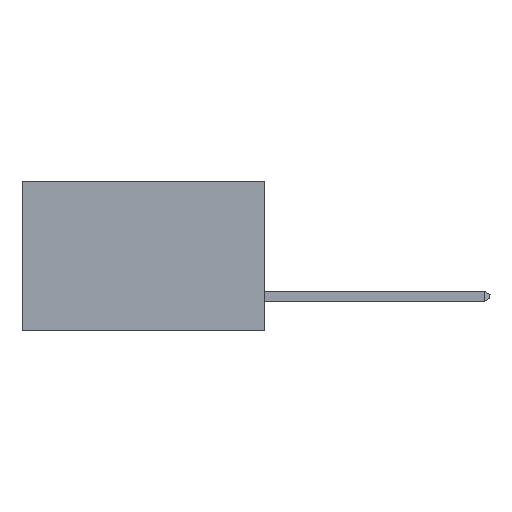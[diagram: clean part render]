
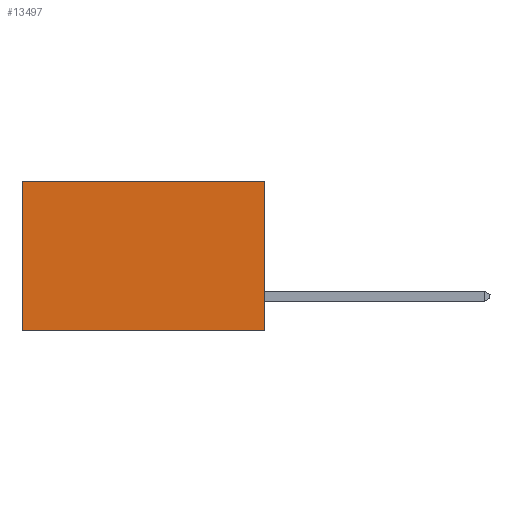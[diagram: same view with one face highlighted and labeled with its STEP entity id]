
A CAD part, left-side view. The second image highlights one B-rep face of the part: STEP entity #13497.
In plain terms, the highlighted planar face has unit normal (-1, 0, 0).
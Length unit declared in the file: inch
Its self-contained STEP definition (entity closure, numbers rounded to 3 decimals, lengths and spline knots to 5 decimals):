
#767 = VECTOR ( 'NONE', #15023, 39.37008 ) ;
#2367 = EDGE_CURVE ( 'NONE', #17266, #6237, #12811, .T. ) ;
#2376 = DIRECTION ( 'NONE',  ( 0., 0., -1. ) ) ;
#2412 = EDGE_CURVE ( 'NONE', #11081, #6237, #20683, .T. ) ;
#2813 = VERTEX_POINT ( 'NONE', #7000 ) ;
#3855 = CARTESIAN_POINT ( 'NONE',  ( 0.298, 0., 0. ) ) ;
#5524 = VECTOR ( 'NONE', #17310, 39.37008 ) ;
#5639 = CARTESIAN_POINT ( 'NONE',  ( 0.298, 0., 0. ) ) ;
#6237 = VERTEX_POINT ( 'NONE', #21857 ) ;
#6766 = EDGE_CURVE ( 'NONE', #2813, #17266, #20500, .T. ) ;
#7000 = CARTESIAN_POINT ( 'NONE',  ( 0.298, 0., 0. ) ) ;
#7264 = VECTOR ( 'NONE', #2376, 39.37008 ) ;
#7351 = EDGE_LOOP ( 'NONE', ( #19851, #17341, #23448, #23607 ) ) ;
#7435 = CARTESIAN_POINT ( 'NONE',  ( 0.298, 0.6, 0. ) ) ;
#11081 = VERTEX_POINT ( 'NONE', #12309 ) ;
#12309 = CARTESIAN_POINT ( 'NONE',  ( 0.298, 0., -0.37 ) ) ;
#12811 = LINE ( 'NONE', #7435, #767 ) ;
#13497 = ADVANCED_FACE ( 'NONE', ( #16140 ), #19964, .F. ) ;
#13769 = DIRECTION ( 'NONE',  ( 0., 1., 0. ) ) ;
#14252 = EDGE_CURVE ( 'NONE', #2813, #11081, #20737, .T. ) ;
#14852 = VECTOR ( 'NONE', #13769, 39.37008 ) ;
#14979 = CARTESIAN_POINT ( 'NONE',  ( 0.298, 0.6, 0. ) ) ;
#15023 = DIRECTION ( 'NONE',  ( 0., 0., -1. ) ) ;
#16140 = FACE_OUTER_BOUND ( 'NONE', #7351, .T. ) ;
#16611 = DIRECTION ( 'NONE',  ( 1., 0., 0. ) ) ;
#17266 = VERTEX_POINT ( 'NONE', #14979 ) ;
#17310 = DIRECTION ( 'NONE',  ( 0., 1., 0. ) ) ;
#17341 = ORIENTED_EDGE ( 'NONE', *, *, #2412, .F. ) ;
#17658 = CARTESIAN_POINT ( 'NONE',  ( 0.298, 0., -0.37 ) ) ;
#19851 = ORIENTED_EDGE ( 'NONE', *, *, #2367, .T. ) ;
#19964 = PLANE ( 'NONE',  #21084 ) ;
#20442 = CARTESIAN_POINT ( 'NONE',  ( 0.298, 0., 0. ) ) ;
#20500 = LINE ( 'NONE', #5639, #5524 ) ;
#20683 = LINE ( 'NONE', #17658, #14852 ) ;
#20737 = LINE ( 'NONE', #3855, #7264 ) ;
#21084 = AXIS2_PLACEMENT_3D ( 'NONE', #20442, #16611, #23594 ) ;
#21857 = CARTESIAN_POINT ( 'NONE',  ( 0.298, 0.6, -0.37 ) ) ;
#23448 = ORIENTED_EDGE ( 'NONE', *, *, #14252, .F. ) ;
#23594 = DIRECTION ( 'NONE',  ( 0., 0., -1. ) ) ;
#23607 = ORIENTED_EDGE ( 'NONE', *, *, #6766, .T. ) ;
